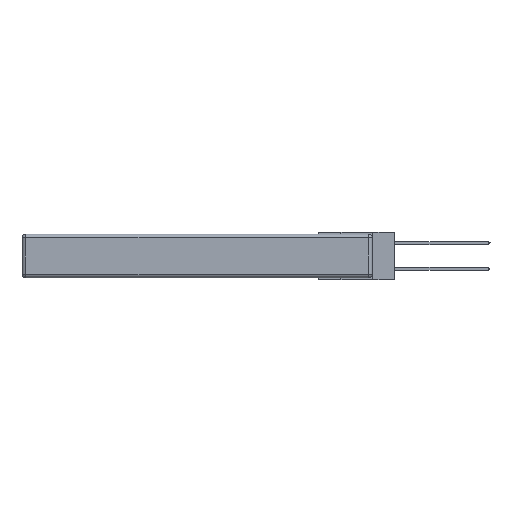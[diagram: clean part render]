
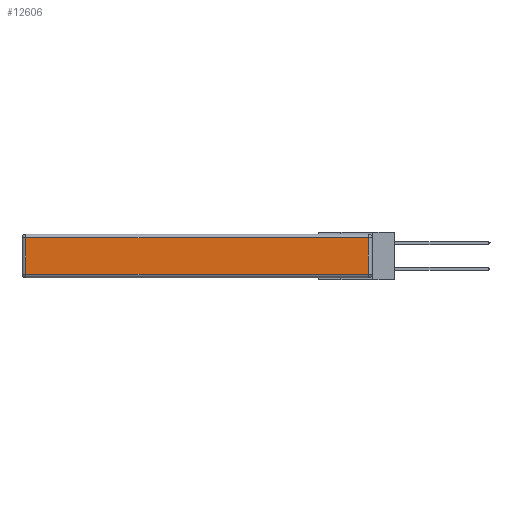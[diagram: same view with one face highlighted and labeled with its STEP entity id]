
A CAD part, left-side view. The second image highlights one B-rep face of the part: STEP entity #12606.
In plain terms, the highlighted planar face has unit normal (-1, 0, 0).
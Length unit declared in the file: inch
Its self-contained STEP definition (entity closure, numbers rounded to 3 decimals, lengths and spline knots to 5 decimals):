
#158 = ORIENTED_EDGE ( 'NONE', *, *, #3304, .T. ) ;
#664 = ORIENTED_EDGE ( 'NONE', *, *, #14805, .T. ) ;
#969 = CARTESIAN_POINT ( 'NONE',  ( 0., 0., -0.313 ) ) ;
#1019 = LINE ( 'NONE', #7627, #4429 ) ;
#2228 = DIRECTION ( 'NONE',  ( 0., -1., 0. ) ) ;
#2402 = FACE_OUTER_BOUND ( 'NONE', #13137, .T. ) ;
#3065 = DIRECTION ( 'NONE',  ( -1., 0., 0. ) ) ;
#3292 = CARTESIAN_POINT ( 'NONE',  ( 0., 0.03, -0.03 ) ) ;
#3304 = EDGE_CURVE ( 'NONE', #14052, #6756, #3638, .T. ) ;
#3355 = VERTEX_POINT ( 'NONE', #6542 ) ;
#3638 = LINE ( 'NONE', #11646, #13980 ) ;
#4429 = VECTOR ( 'NONE', #12169, 39.37008 ) ;
#6052 = ORIENTED_EDGE ( 'NONE', *, *, #9551, .T. ) ;
#6470 = LINE ( 'NONE', #8546, #9825 ) ;
#6478 = PLANE ( 'NONE',  #10869 ) ;
#6542 = CARTESIAN_POINT ( 'NONE',  ( 0., 2.72, -0.313 ) ) ;
#6756 = VERTEX_POINT ( 'NONE', #3292 ) ;
#6860 = VECTOR ( 'NONE', #2228, 39.37008 ) ;
#7627 = CARTESIAN_POINT ( 'NONE',  ( 0., 2.75, -0.03 ) ) ;
#8546 = CARTESIAN_POINT ( 'NONE',  ( 0., 2.72, -0.343 ) ) ;
#9317 = LINE ( 'NONE', #969, #6860 ) ;
#9551 = EDGE_CURVE ( 'NONE', #3355, #14052, #9317, .T. ) ;
#9825 = VECTOR ( 'NONE', #12044, 39.37008 ) ;
#9882 = CARTESIAN_POINT ( 'NONE',  ( 0., 0., -0.343 ) ) ;
#10636 = EDGE_CURVE ( 'NONE', #6756, #13612, #1019, .T. ) ;
#10779 = DIRECTION ( 'NONE',  ( 0., 0., 1. ) ) ;
#10869 = AXIS2_PLACEMENT_3D ( 'NONE', #9882, #3065, #13219 ) ;
#11646 = CARTESIAN_POINT ( 'NONE',  ( 0., 0.03, -0.343 ) ) ;
#12044 = DIRECTION ( 'NONE',  ( 0., 0., -1. ) ) ;
#12169 = DIRECTION ( 'NONE',  ( 0., 1., 0. ) ) ;
#12503 = ORIENTED_EDGE ( 'NONE', *, *, #10636, .T. ) ;
#12606 = ADVANCED_FACE ( 'NONE', ( #2402 ), #6478, .T. ) ;
#13137 = EDGE_LOOP ( 'NONE', ( #6052, #158, #12503, #664 ) ) ;
#13219 = DIRECTION ( 'NONE',  ( 0., 0., 1. ) ) ;
#13612 = VERTEX_POINT ( 'NONE', #14253 ) ;
#13838 = CARTESIAN_POINT ( 'NONE',  ( 0., 0.03, -0.313 ) ) ;
#13980 = VECTOR ( 'NONE', #10779, 39.37008 ) ;
#14052 = VERTEX_POINT ( 'NONE', #13838 ) ;
#14253 = CARTESIAN_POINT ( 'NONE',  ( 0., 2.72, -0.03 ) ) ;
#14805 = EDGE_CURVE ( 'NONE', #13612, #3355, #6470, .T. ) ;
